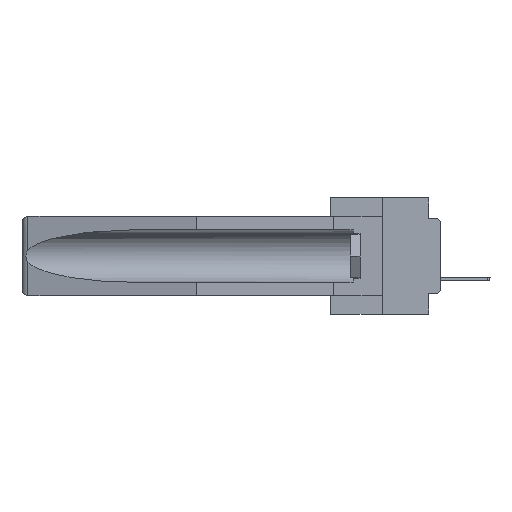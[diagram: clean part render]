
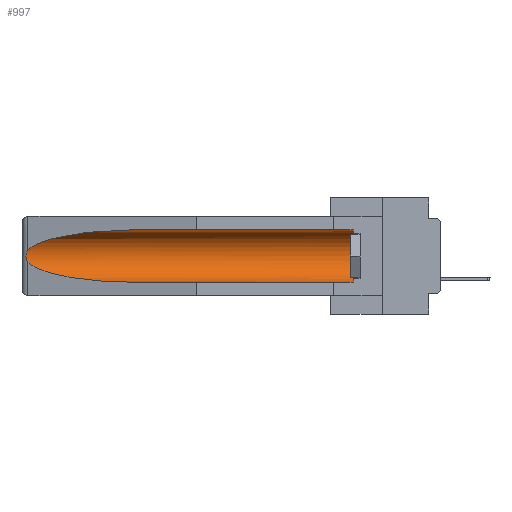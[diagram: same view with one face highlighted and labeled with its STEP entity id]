
A CAD part, left-side view. The second image highlights one B-rep face of the part: STEP entity #997.
In plain terms, the highlighted cylindrical face has radius 2.857 mm (diameter 5.715 mm), a partial arc.
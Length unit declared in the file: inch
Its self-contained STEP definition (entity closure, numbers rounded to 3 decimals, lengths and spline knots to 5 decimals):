
#162 = LINE ( 'NONE', #31660, #7610 ) ;
#192 = CARTESIAN_POINT ( 'NONE',  ( 0.26537, 1.52718, -0.14972 ) ) ;
#997 = ADVANCED_FACE ( 'NONE', ( #19648 ), #30144, .F. ) ;
#1884 = EDGE_CURVE ( 'NONE', #15378, #14309, #22033, .T. ) ;
#2132 = CARTESIAN_POINT ( 'NONE',  ( 0.26537, 1.52718, -0.19328 ) ) ;
#2480 = CARTESIAN_POINT ( 'NONE',  ( 0.21114, 1.30732, -0.284 ) ) ;
#2997 = CARTESIAN_POINT ( 'NONE',  ( 0.155, 0.126, -0.284 ) ) ;
#3972 = DIRECTION ( 'NONE',  ( 0., 1., 0. ) ) ;
#4056 = VERTEX_POINT ( 'NONE', #10825 ) ;
#4727 = EDGE_CURVE ( 'NONE', #27034, #4056, #21465, .T. ) ;
#5394 = CARTESIAN_POINT ( 'NONE',  ( 0.26655, 1.53094, -0.18657 ) ) ;
#6156 = CARTESIAN_POINT ( 'NONE',  ( 0.21114, 1.30732, -0.059 ) ) ;
#6976 = CARTESIAN_POINT ( 'NONE',  ( 0.155, 1.07973, -0.284 ) ) ;
#7395 = VERTEX_POINT ( 'NONE', #24880 ) ;
#7492 = VERTEX_POINT ( 'NONE', #6976 ) ;
#7610 = VECTOR ( 'NONE', #10507, 39.37008 ) ;
#7644 = CARTESIAN_POINT ( 'NONE',  ( 0.26654, 1.53092, -0.15636 ) ) ;
#7733 = ORIENTED_EDGE ( 'NONE', *, *, #15106, .T. ) ;
#7987 = CARTESIAN_POINT ( 'NONE',  ( 0.26537, 1.52718, -0.19328 ) ) ;
#9872 = DIRECTION ( 'NONE',  ( 0., 0., 1. ) ) ;
#10027 = EDGE_CURVE ( 'NONE', #15378, #7492, #33794, .T. ) ;
#10057 = CARTESIAN_POINT ( 'NONE',  ( 0.155, -0.30754, -0.284 ) ) ;
#10507 = DIRECTION ( 'NONE',  ( 0., 1., 0. ) ) ;
#10566 = CARTESIAN_POINT ( 'NONE',  ( 0.26597, 1.5296, -0.19026 ) ) ;
#10825 = CARTESIAN_POINT ( 'NONE',  ( 0.26537, 1.52718, -0.19328 ) ) ;
#11084 = AXIS2_PLACEMENT_3D ( 'NONE', #27557, #3972, #12755 ) ;
#12755 = DIRECTION ( 'NONE',  ( 0., 0., 1. ) ) ;
#13147 = CARTESIAN_POINT ( 'NONE',  ( 0.2675, 1.53308, -0.16763 ) ) ;
#13677 = CARTESIAN_POINT ( 'NONE',  ( 0.155, 0.126, -0.059 ) ) ;
#14309 = VERTEX_POINT ( 'NONE', #13677 ) ;
#15035 = CARTESIAN_POINT ( 'NONE',  ( 0.155, 0.126, -0.1715 ) ) ;
#15106 = EDGE_CURVE ( 'NONE', #7395, #27034, #20666, .T. ) ;
#15378 = VERTEX_POINT ( 'NONE', #2997 ) ;
#15736 = CARTESIAN_POINT ( 'NONE',  ( 0.2673, 1.5327, -0.16383 ) ) ;
#16659 = CARTESIAN_POINT ( 'NONE',  ( 0.25451, 1.48313, -0.09465 ) ) ;
#18576 = EDGE_CURVE ( 'NONE', #4056, #7492, #26581, .T. ) ;
#19600 = EDGE_CURVE ( 'NONE', #14309, #7395, #162, .T. ) ;
#19648 = FACE_OUTER_BOUND ( 'NONE', #33141, .T. ) ;
#20666 =( BOUNDED_CURVE ( )  B_SPLINE_CURVE ( 3, ( #29736, #6156, #16659, #30241 ),
 .UNSPECIFIED., .F., .T. ) 
 B_SPLINE_CURVE_WITH_KNOTS ( ( 4, 4 ),
 ( 4.71239, 6.08839 ),
 .UNSPECIFIED. ) 
 CURVE ( )  GEOMETRIC_REPRESENTATION_ITEM ( )  RATIONAL_B_SPLINE_CURVE ( ( 1., 0.848, 0.848, 1. ) ) 
 REPRESENTATION_ITEM ( '' )  );
#21465 = B_SPLINE_CURVE_WITH_KNOTS ( 'NONE', 3,
 ( #23483, #31893, #7644, #15736, #13147, #28634, #23645, #5394, #10566, #7987 ),
 .UNSPECIFIED., .F., .F.,
 ( 4, 2, 2, 2, 4 ),
 ( 0., 0.00029, 0.00058, 0.00087, 0.00117 ),
 .UNSPECIFIED. ) ;
#22033 = CIRCLE ( 'NONE', #33011, 0.1125 ) ;
#22223 = ORIENTED_EDGE ( 'NONE', *, *, #1884, .T. ) ;
#23483 = CARTESIAN_POINT ( 'NONE',  ( 0.26537, 1.52718, -0.14972 ) ) ;
#23645 = CARTESIAN_POINT ( 'NONE',  ( 0.2673, 1.53269, -0.17917 ) ) ;
#23648 = DIRECTION ( 'NONE',  ( 0., 1., 0. ) ) ;
#23668 = VECTOR ( 'NONE', #23648, 39.37008 ) ;
#24880 = CARTESIAN_POINT ( 'NONE',  ( 0.155, 1.07973, -0.059 ) ) ;
#25529 = DIRECTION ( 'NONE',  ( 0., -1., 0. ) ) ;
#26565 = ORIENTED_EDGE ( 'NONE', *, *, #4727, .T. ) ;
#26581 =( BOUNDED_CURVE ( )  B_SPLINE_CURVE ( 3, ( #2132, #30904, #2480, #31073 ),
 .UNSPECIFIED., .F., .F. ) 
 B_SPLINE_CURVE_WITH_KNOTS ( ( 4, 4 ),
 ( 0.1948, 1.5708 ),
 .UNSPECIFIED. ) 
 CURVE ( )  GEOMETRIC_REPRESENTATION_ITEM ( )  RATIONAL_B_SPLINE_CURVE ( ( 1., 0.848, 0.848, 1. ) ) 
 REPRESENTATION_ITEM ( '' )  );
#27034 = VERTEX_POINT ( 'NONE', #192 ) ;
#27557 = CARTESIAN_POINT ( 'NONE',  ( 0.155, -0.30754, -0.1715 ) ) ;
#27926 = ORIENTED_EDGE ( 'NONE', *, *, #18576, .T. ) ;
#28450 = ORIENTED_EDGE ( 'NONE', *, *, #10027, .F. ) ;
#28634 = CARTESIAN_POINT ( 'NONE',  ( 0.2675, 1.53308, -0.17534 ) ) ;
#29736 = CARTESIAN_POINT ( 'NONE',  ( 0.155, 1.07973, -0.059 ) ) ;
#29982 = ORIENTED_EDGE ( 'NONE', *, *, #19600, .T. ) ;
#30144 = CYLINDRICAL_SURFACE ( 'NONE', #11084, 0.1125 ) ;
#30241 = CARTESIAN_POINT ( 'NONE',  ( 0.26537, 1.52718, -0.14972 ) ) ;
#30904 = CARTESIAN_POINT ( 'NONE',  ( 0.25451, 1.48313, -0.24835 ) ) ;
#31073 = CARTESIAN_POINT ( 'NONE',  ( 0.155, 1.07973, -0.284 ) ) ;
#31660 = CARTESIAN_POINT ( 'NONE',  ( 0.155, -0.30754, -0.059 ) ) ;
#31893 = CARTESIAN_POINT ( 'NONE',  ( 0.26597, 1.52961, -0.15275 ) ) ;
#33011 = AXIS2_PLACEMENT_3D ( 'NONE', #15035, #25529, #9872 ) ;
#33141 = EDGE_LOOP ( 'NONE', ( #7733, #26565, #27926, #28450, #22223, #29982 ) ) ;
#33794 = LINE ( 'NONE', #10057, #23668 ) ;
